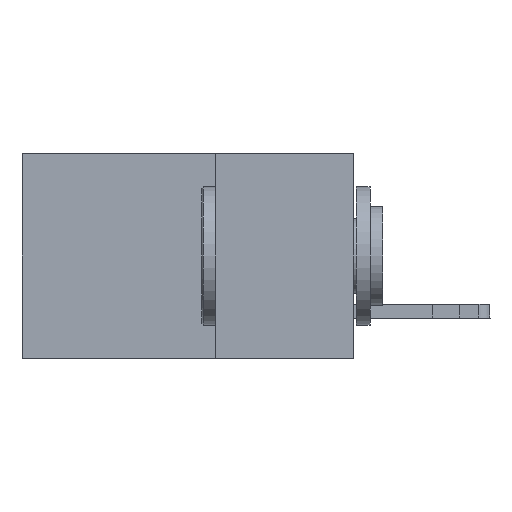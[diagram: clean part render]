
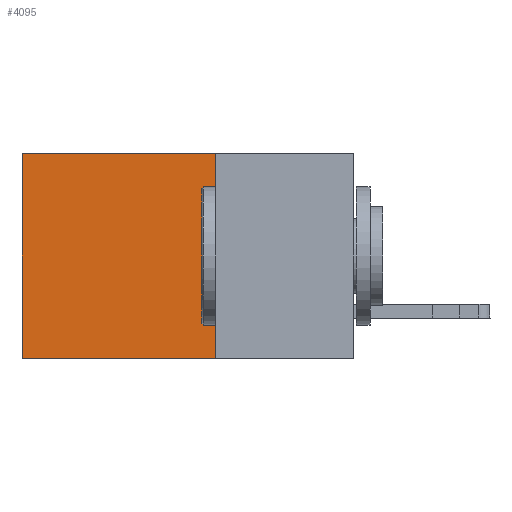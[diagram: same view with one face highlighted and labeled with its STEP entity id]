
A CAD part, left-side view. The second image highlights one B-rep face of the part: STEP entity #4095.
In plain terms, the highlighted planar face has unit normal (-1, 0, 0).
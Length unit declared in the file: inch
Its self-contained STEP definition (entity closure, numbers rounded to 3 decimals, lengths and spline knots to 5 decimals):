
#2008 = ORIENTED_EDGE ( 'NONE', *, *, #4353, .F. ) ;
#2022 = CARTESIAN_POINT ( 'NONE',  ( 0.2875, 0.6, -0.37 ) ) ;
#2556 = EDGE_CURVE ( 'NONE', #10848, #5852, #18967, .T. ) ;
#2670 = DIRECTION ( 'NONE',  ( 1., 0., 0. ) ) ;
#3443 = VECTOR ( 'NONE', #4491, 39.37008 ) ;
#3792 = CARTESIAN_POINT ( 'NONE',  ( 0.2875, 0.6, 0. ) ) ;
#4095 = ADVANCED_FACE ( 'NONE', ( #14409 ), #14552, .F. ) ;
#4240 = DIRECTION ( 'NONE',  ( 0., 1., 0. ) ) ;
#4353 = EDGE_CURVE ( 'NONE', #10442, #20688, #7088, .T. ) ;
#4491 = DIRECTION ( 'NONE',  ( 0., 0., -1. ) ) ;
#4558 = DIRECTION ( 'NONE',  ( 0., 0., -1. ) ) ;
#4745 = VECTOR ( 'NONE', #4240, 39.37008 ) ;
#5852 = VERTEX_POINT ( 'NONE', #8788 ) ;
#7088 = LINE ( 'NONE', #14299, #4745 ) ;
#7428 = ORIENTED_EDGE ( 'NONE', *, *, #2556, .T. ) ;
#7636 = CARTESIAN_POINT ( 'NONE',  ( 0.2875, 0.25, 0. ) ) ;
#7825 = CARTESIAN_POINT ( 'NONE',  ( 0.2875, 0.25, 0. ) ) ;
#7881 = LINE ( 'NONE', #15934, #3443 ) ;
#8091 = AXIS2_PLACEMENT_3D ( 'NONE', #7825, #2670, #4558 ) ;
#8788 = CARTESIAN_POINT ( 'NONE',  ( 0.2875, 0.6, 0. ) ) ;
#9182 = EDGE_CURVE ( 'NONE', #5852, #20688, #18686, .T. ) ;
#9769 = VECTOR ( 'NONE', #15463, 39.37008 ) ;
#10442 = VERTEX_POINT ( 'NONE', #13016 ) ;
#10848 = VERTEX_POINT ( 'NONE', #7636 ) ;
#11318 = EDGE_CURVE ( 'NONE', #10848, #10442, #7881, .T. ) ;
#12733 = ORIENTED_EDGE ( 'NONE', *, *, #9182, .T. ) ;
#13016 = CARTESIAN_POINT ( 'NONE',  ( 0.2875, 0.25, -0.37 ) ) ;
#14175 = ORIENTED_EDGE ( 'NONE', *, *, #11318, .F. ) ;
#14299 = CARTESIAN_POINT ( 'NONE',  ( 0.2875, 0.25, -0.37 ) ) ;
#14409 = FACE_OUTER_BOUND ( 'NONE', #18366, .T. ) ;
#14552 = PLANE ( 'NONE',  #8091 ) ;
#15463 = DIRECTION ( 'NONE',  ( 0., 0., -1. ) ) ;
#15777 = VECTOR ( 'NONE', #16259, 39.37008 ) ;
#15934 = CARTESIAN_POINT ( 'NONE',  ( 0.2875, 0.25, 0. ) ) ;
#16259 = DIRECTION ( 'NONE',  ( 0., 1., 0. ) ) ;
#18366 = EDGE_LOOP ( 'NONE', ( #12733, #2008, #14175, #7428 ) ) ;
#18686 = LINE ( 'NONE', #3792, #9769 ) ;
#18967 = LINE ( 'NONE', #19609, #15777 ) ;
#19609 = CARTESIAN_POINT ( 'NONE',  ( 0.2875, 0.25, 0. ) ) ;
#20688 = VERTEX_POINT ( 'NONE', #2022 ) ;
